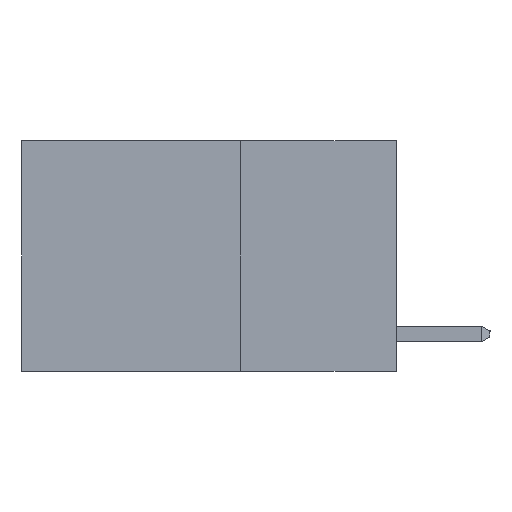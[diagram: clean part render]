
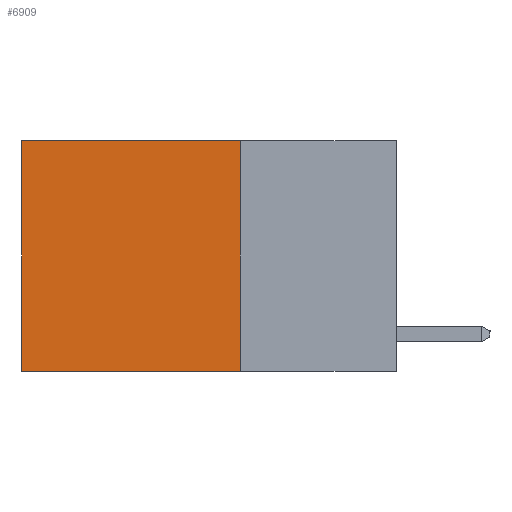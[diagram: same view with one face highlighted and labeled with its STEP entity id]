
A CAD part, left-side view. The second image highlights one B-rep face of the part: STEP entity #6909.
In plain terms, the highlighted planar face has unit normal (-1, 0, 0).
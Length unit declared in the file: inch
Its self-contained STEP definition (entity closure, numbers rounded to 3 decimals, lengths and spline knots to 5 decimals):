
#74 = FACE_OUTER_BOUND ( 'NONE', #10173, .T. ) ;
#674 = CARTESIAN_POINT ( 'NONE',  ( 0.2625, 0.25, -0.37 ) ) ;
#682 = AXIS2_PLACEMENT_3D ( 'NONE', #3946, #12774, #5227 ) ;
#700 = CARTESIAN_POINT ( 'NONE',  ( 0.2625, 0.6, 0. ) ) ;
#2048 = DIRECTION ( 'NONE',  ( 0., 1., 0. ) ) ;
#2920 = VECTOR ( 'NONE', #2048, 39.37008 ) ;
#3041 = EDGE_CURVE ( 'NONE', #10321, #12436, #3457, .T. ) ;
#3214 = CARTESIAN_POINT ( 'NONE',  ( 0.2625, 0.6, 0. ) ) ;
#3457 = LINE ( 'NONE', #16270, #9439 ) ;
#3685 = CARTESIAN_POINT ( 'NONE',  ( 0.2625, 0.25, -0.37 ) ) ;
#3946 = CARTESIAN_POINT ( 'NONE',  ( 0.2625, 0.25, 0. ) ) ;
#4525 = DIRECTION ( 'NONE',  ( 0., 0., -1. ) ) ;
#4875 = EDGE_CURVE ( 'NONE', #12436, #7795, #5469, .T. ) ;
#5116 = PLANE ( 'NONE',  #682 ) ;
#5227 = DIRECTION ( 'NONE',  ( 0., 0., -1. ) ) ;
#5367 = ORIENTED_EDGE ( 'NONE', *, *, #10088, .F. ) ;
#5401 = ORIENTED_EDGE ( 'NONE', *, *, #3041, .T. ) ;
#5469 = LINE ( 'NONE', #700, #15046 ) ;
#6909 = ADVANCED_FACE ( 'NONE', ( #74 ), #5116, .F. ) ;
#7795 = VERTEX_POINT ( 'NONE', #9603 ) ;
#7867 = VECTOR ( 'NONE', #10330, 39.37008 ) ;
#8671 = VERTEX_POINT ( 'NONE', #3685 ) ;
#8851 = CARTESIAN_POINT ( 'NONE',  ( 0.2625, 0.25, 0. ) ) ;
#9076 = CARTESIAN_POINT ( 'NONE',  ( 0.2625, 0.25, 0. ) ) ;
#9281 = ORIENTED_EDGE ( 'NONE', *, *, #4875, .T. ) ;
#9439 = VECTOR ( 'NONE', #10199, 39.37008 ) ;
#9523 = ORIENTED_EDGE ( 'NONE', *, *, #10425, .F. ) ;
#9603 = CARTESIAN_POINT ( 'NONE',  ( 0.2625, 0.6, -0.37 ) ) ;
#9694 = LINE ( 'NONE', #674, #2920 ) ;
#10088 = EDGE_CURVE ( 'NONE', #8671, #7795, #9694, .T. ) ;
#10173 = EDGE_LOOP ( 'NONE', ( #9281, #5367, #9523, #5401 ) ) ;
#10199 = DIRECTION ( 'NONE',  ( 0., 1., 0. ) ) ;
#10321 = VERTEX_POINT ( 'NONE', #8851 ) ;
#10330 = DIRECTION ( 'NONE',  ( 0., 0., -1. ) ) ;
#10425 = EDGE_CURVE ( 'NONE', #10321, #8671, #10857, .T. ) ;
#10857 = LINE ( 'NONE', #9076, #7867 ) ;
#12436 = VERTEX_POINT ( 'NONE', #3214 ) ;
#12774 = DIRECTION ( 'NONE',  ( 1., 0., 0. ) ) ;
#15046 = VECTOR ( 'NONE', #4525, 39.37008 ) ;
#16270 = CARTESIAN_POINT ( 'NONE',  ( 0.2625, 0.25, 0. ) ) ;
